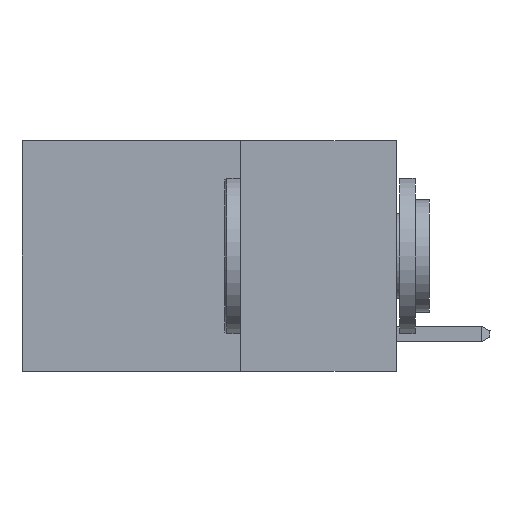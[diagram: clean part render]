
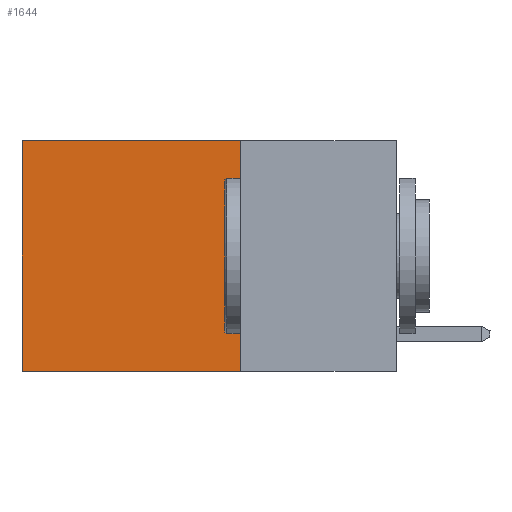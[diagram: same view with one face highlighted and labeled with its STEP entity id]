
A CAD part, left-side view. The second image highlights one B-rep face of the part: STEP entity #1644.
In plain terms, the highlighted planar face has unit normal (-1, 0, 0).
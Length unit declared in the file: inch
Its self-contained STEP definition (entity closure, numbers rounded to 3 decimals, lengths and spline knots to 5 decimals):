
#204 = LINE ( 'NONE', #1103, #16459 ) ;
#1103 = CARTESIAN_POINT ( 'NONE',  ( 0.2625, 0.25, -0.37 ) ) ;
#1570 = DIRECTION ( 'NONE',  ( 0., 0., -1. ) ) ;
#1603 = CARTESIAN_POINT ( 'NONE',  ( 0.2625, 0.6, 0. ) ) ;
#1644 = ADVANCED_FACE ( 'NONE', ( #11588 ), #15844, .F. ) ;
#3872 = DIRECTION ( 'NONE',  ( 0., 0., -1. ) ) ;
#4106 = ORIENTED_EDGE ( 'NONE', *, *, #14048, .F. ) ;
#4308 = VERTEX_POINT ( 'NONE', #1603 ) ;
#4463 = CARTESIAN_POINT ( 'NONE',  ( 0.2625, 0.25, 0. ) ) ;
#4941 = ORIENTED_EDGE ( 'NONE', *, *, #8650, .F. ) ;
#6777 = DIRECTION ( 'NONE',  ( 1., 0., 0. ) ) ;
#6936 = EDGE_LOOP ( 'NONE', ( #9831, #4941, #4106, #10160 ) ) ;
#7337 = CARTESIAN_POINT ( 'NONE',  ( 0.2625, 0.25, 0. ) ) ;
#8650 = EDGE_CURVE ( 'NONE', #10690, #12641, #204, .T. ) ;
#8777 = CARTESIAN_POINT ( 'NONE',  ( 0.2625, 0.6, -0.37 ) ) ;
#9729 = CARTESIAN_POINT ( 'NONE',  ( 0.2625, 0.25, 0. ) ) ;
#9831 = ORIENTED_EDGE ( 'NONE', *, *, #12599, .T. ) ;
#9956 = LINE ( 'NONE', #12007, #15127 ) ;
#10160 = ORIENTED_EDGE ( 'NONE', *, *, #17820, .T. ) ;
#10690 = VERTEX_POINT ( 'NONE', #16355 ) ;
#10708 = VECTOR ( 'NONE', #17924, 39.37008 ) ;
#11588 = FACE_OUTER_BOUND ( 'NONE', #6936, .T. ) ;
#11848 = DIRECTION ( 'NONE',  ( 0., 0., -1. ) ) ;
#12007 = CARTESIAN_POINT ( 'NONE',  ( 0.2625, 0.25, 0. ) ) ;
#12599 = EDGE_CURVE ( 'NONE', #4308, #12641, #16619, .T. ) ;
#12641 = VERTEX_POINT ( 'NONE', #8777 ) ;
#12758 = AXIS2_PLACEMENT_3D ( 'NONE', #9729, #6777, #3872 ) ;
#14048 = EDGE_CURVE ( 'NONE', #18086, #10690, #9956, .T. ) ;
#15127 = VECTOR ( 'NONE', #1570, 39.37008 ) ;
#15844 = PLANE ( 'NONE',  #12758 ) ;
#16355 = CARTESIAN_POINT ( 'NONE',  ( 0.2625, 0.25, -0.37 ) ) ;
#16459 = VECTOR ( 'NONE', #18286, 39.37008 ) ;
#16619 = LINE ( 'NONE', #19376, #17070 ) ;
#17047 = LINE ( 'NONE', #7337, #10708 ) ;
#17070 = VECTOR ( 'NONE', #11848, 39.37008 ) ;
#17820 = EDGE_CURVE ( 'NONE', #18086, #4308, #17047, .T. ) ;
#17924 = DIRECTION ( 'NONE',  ( 0., 1., 0. ) ) ;
#18086 = VERTEX_POINT ( 'NONE', #4463 ) ;
#18286 = DIRECTION ( 'NONE',  ( 0., 1., 0. ) ) ;
#19376 = CARTESIAN_POINT ( 'NONE',  ( 0.2625, 0.6, 0. ) ) ;
